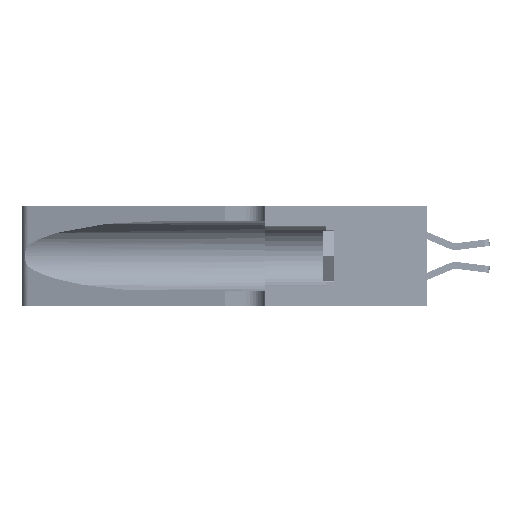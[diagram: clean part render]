
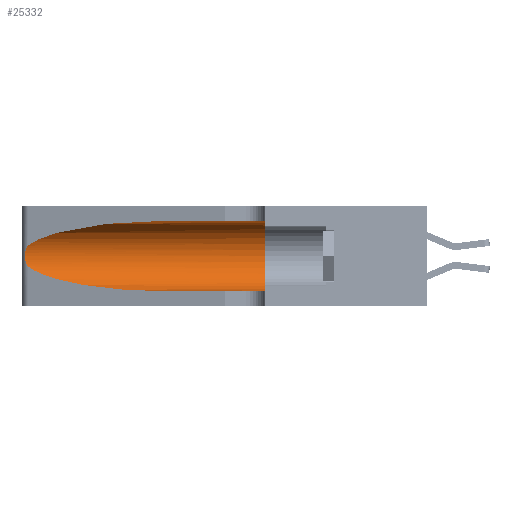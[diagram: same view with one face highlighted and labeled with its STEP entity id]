
A CAD part, left-side view. The second image highlights one B-rep face of the part: STEP entity #25332.
In plain terms, the highlighted cylindrical face has radius 3.308 mm (diameter 6.617 mm), a partial arc.
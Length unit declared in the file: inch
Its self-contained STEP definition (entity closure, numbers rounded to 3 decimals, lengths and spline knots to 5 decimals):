
#65 = VERTEX_POINT ( 'NONE', #37583 ) ;
#91 = ORIENTED_EDGE ( 'NONE', *, *, #30386, .F. ) ;
#122 = ORIENTED_EDGE ( 'NONE', *, *, #450, .F. ) ;
#450 = EDGE_CURVE ( 'NONE', #18315, #31167, #6648, .T. ) ;
#1387 = VERTEX_POINT ( 'NONE', #17262 ) ;
#1944 = EDGE_CURVE ( 'NONE', #1387, #38418, #49457, .T. ) ;
#2798 = CARTESIAN_POINT ( 'NONE',  ( 0.25787, 1.23484, 0.2124 ) ) ;
#4171 = CARTESIAN_POINT ( 'NONE',  ( 0.1305, 0.72297, 0.31525 ) ) ;
#4606 = LINE ( 'NONE', #4955, #28671 ) ;
#4955 = CARTESIAN_POINT ( 'NONE',  ( 0.1305, 1.61858, 0.05475 ) ) ;
#6153 = CARTESIAN_POINT ( 'NONE',  ( 0.25487, 1.22718, 0.14631 ) ) ;
#6317 = CARTESIAN_POINT ( 'NONE',  ( 0.26075, 1.23896, 0.19203 ) ) ;
#6648 = CIRCLE ( 'NONE', #7996, 0.13025 ) ;
#6945 =( BOUNDED_CURVE ( )  B_SPLINE_CURVE ( 3, ( #4171, #11710, #12040, #30737 ),
 .UNSPECIFIED., .F., .T. ) 
 B_SPLINE_CURVE_WITH_KNOTS ( ( 4, 4 ),
 ( 1.5708, 2.84003 ),
 .UNSPECIFIED. ) 
 CURVE ( )  GEOMETRIC_REPRESENTATION_ITEM ( )  RATIONAL_B_SPLINE_CURVE ( ( 1., 0.87, 0.87, 1. ) ) 
 REPRESENTATION_ITEM ( '' )  );
#7996 = AXIS2_PLACEMENT_3D ( 'NONE', #35872, #12263, #24031 ) ;
#8115 = CARTESIAN_POINT ( 'NONE',  ( 0.2373, 1.15595, 0.08982 ) ) ;
#8628 = DIRECTION ( 'NONE',  ( 0., -1., 0. ) ) ;
#8794 = ORIENTED_EDGE ( 'NONE', *, *, #1944, .T. ) ;
#9711 = CARTESIAN_POINT ( 'NONE',  ( 0.1305, 0.72297, 0.05475 ) ) ;
#11082 = DIRECTION ( 'NONE',  ( 0., 0., -1. ) ) ;
#11710 = CARTESIAN_POINT ( 'NONE',  ( 0.18966, 0.96281, 0.31525 ) ) ;
#11839 = CARTESIAN_POINT ( 'NONE',  ( 0.1305, 0.72297, 0.05475 ) ) ;
#11999 = CARTESIAN_POINT ( 'NONE',  ( 0.18966, 0.96281, 0.05475 ) ) ;
#12040 = CARTESIAN_POINT ( 'NONE',  ( 0.2373, 1.15595, 0.28018 ) ) ;
#12175 = CARTESIAN_POINT ( 'NONE',  ( 0.25487, 1.22718, 0.14631 ) ) ;
#12263 = DIRECTION ( 'NONE',  ( 0., 1., 0. ) ) ;
#14239 = CARTESIAN_POINT ( 'NONE',  ( 0.26017, 1.23833, 0.17102 ) ) ;
#14397 = CARTESIAN_POINT ( 'NONE',  ( 0.25854, 1.2359, 0.20912 ) ) ;
#17262 = CARTESIAN_POINT ( 'NONE',  ( 0.25487, 1.22718, 0.22369 ) ) ;
#17973 = CARTESIAN_POINT ( 'NONE',  ( 0.25789, 1.23486, 0.15765 ) ) ;
#18315 = VERTEX_POINT ( 'NONE', #26518 ) ;
#18375 = CARTESIAN_POINT ( 'NONE',  ( 0.1305, 1.61858, 0.185 ) ) ;
#21993 = CARTESIAN_POINT ( 'NONE',  ( 0.25487, 1.22718, 0.22369 ) ) ;
#22223 = ORIENTED_EDGE ( 'NONE', *, *, #39863, .T. ) ;
#22707 = CARTESIAN_POINT ( 'NONE',  ( 0.1305, 1.61858, 0.31525 ) ) ;
#24031 = DIRECTION ( 'NONE',  ( 0., 0., 1. ) ) ;
#25332 = ADVANCED_FACE ( 'NONE', ( #37245 ), #42649, .F. ) ;
#26238 = EDGE_CURVE ( 'NONE', #49052, #31167, #4606, .T. ) ;
#26518 = CARTESIAN_POINT ( 'NONE',  ( 0.1305, 0.35, 0.31525 ) ) ;
#28671 = VECTOR ( 'NONE', #8628, 39.37008 ) ;
#30258 = DIRECTION ( 'NONE',  ( 0., -1., 0. ) ) ;
#30386 = EDGE_CURVE ( 'NONE', #65, #18315, #49085, .T. ) ;
#30737 = CARTESIAN_POINT ( 'NONE',  ( 0.25487, 1.22718, 0.22369 ) ) ;
#30755 = AXIS2_PLACEMENT_3D ( 'NONE', #18375, #30258, #11082 ) ;
#31167 = VERTEX_POINT ( 'NONE', #33328 ) ;
#33328 = CARTESIAN_POINT ( 'NONE',  ( 0.1305, 0.35, 0.05475 ) ) ;
#33840 = EDGE_LOOP ( 'NONE', ( #43956, #8794, #22223, #42740, #122, #91 ) ) ;
#35872 = CARTESIAN_POINT ( 'NONE',  ( 0.1305, 0.35, 0.185 ) ) ;
#36797 = CARTESIAN_POINT ( 'NONE',  ( 0.25856, 1.23593, 0.16098 ) ) ;
#37140 = CARTESIAN_POINT ( 'NONE',  ( 0.25555, 1.22993, 0.14849 ) ) ;
#37245 = FACE_OUTER_BOUND ( 'NONE', #33840, .T. ) ;
#37293 = CARTESIAN_POINT ( 'NONE',  ( 0.26075, 1.23896, 0.178 ) ) ;
#37461 = CARTESIAN_POINT ( 'NONE',  ( 0.25639, 1.23184, 0.21858 ) ) ;
#37583 = CARTESIAN_POINT ( 'NONE',  ( 0.1305, 0.72297, 0.31525 ) ) ;
#37740 = CARTESIAN_POINT ( 'NONE',  ( 0.25487, 1.22718, 0.14631 ) ) ;
#38418 = VERTEX_POINT ( 'NONE', #37740 ) ;
#39051 =( BOUNDED_CURVE ( )  B_SPLINE_CURVE ( 3, ( #12175, #8115, #11999, #11839 ),
 .UNSPECIFIED., .F., .T. ) 
 B_SPLINE_CURVE_WITH_KNOTS ( ( 4, 4 ),
 ( 3.44316, 4.71239 ),
 .UNSPECIFIED. ) 
 CURVE ( )  GEOMETRIC_REPRESENTATION_ITEM ( )  RATIONAL_B_SPLINE_CURVE ( ( 1., 0.87, 0.87, 1. ) ) 
 REPRESENTATION_ITEM ( '' )  );
#39863 = EDGE_CURVE ( 'NONE', #38418, #49052, #39051, .T. ) ;
#40777 = VECTOR ( 'NONE', #49206, 39.37008 ) ;
#41175 = CARTESIAN_POINT ( 'NONE',  ( 0.25639, 1.23186, 0.15144 ) ) ;
#42649 = CYLINDRICAL_SURFACE ( 'NONE', #30755, 0.13025 ) ;
#42740 = ORIENTED_EDGE ( 'NONE', *, *, #26238, .T. ) ;
#43956 = ORIENTED_EDGE ( 'NONE', *, *, #47288, .T. ) ;
#47288 = EDGE_CURVE ( 'NONE', #65, #1387, #6945, .T. ) ;
#48510 = CARTESIAN_POINT ( 'NONE',  ( 0.26018, 1.23835, 0.19895 ) ) ;
#48835 = CARTESIAN_POINT ( 'NONE',  ( 0.25555, 1.22994, 0.2215 ) ) ;
#49052 = VERTEX_POINT ( 'NONE', #9711 ) ;
#49085 = LINE ( 'NONE', #22707, #40777 ) ;
#49206 = DIRECTION ( 'NONE',  ( 0., -1., 0. ) ) ;
#49457 = B_SPLINE_CURVE_WITH_KNOTS ( 'NONE', 3,
 ( #21993, #48835, #37461, #2798, #14397, #48510, #6317, #37293, #14239, #36797, #17973, #41175, #37140, #6153 ),
 .UNSPECIFIED., .F., .F.,
 ( 4, 2, 2, 2, 2, 2, 4 ),
 ( 0., 0.00027, 0.00053, 0.00107, 0.0016, 0.00187, 0.00214 ),
 .UNSPECIFIED. ) ;
